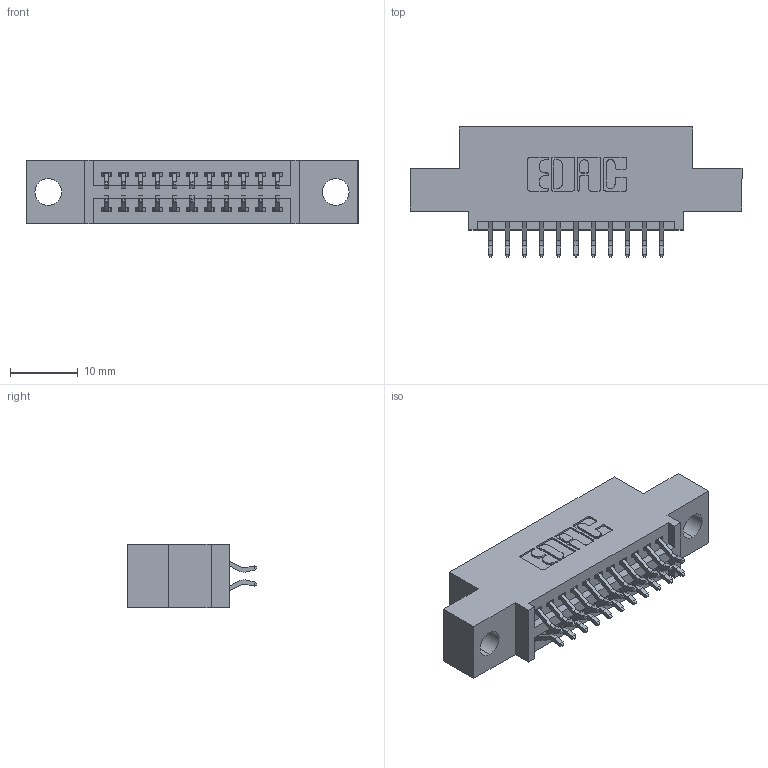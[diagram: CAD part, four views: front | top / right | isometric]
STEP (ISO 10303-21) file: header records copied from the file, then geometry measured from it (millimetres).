
FILE_DESCRIPTION (( 'STEP AP203' ), '1' );
FILE_NAME ('395-022-556-504.STEP', '2021-06-16T18:59:09', ( '' ), ( '' ), 'SwSTEP 2.0', 'SolidWorks 2020', '' );
FILE_SCHEMA (( 'CONFIG_CONTROL_DESIGN' ));
Length unit declared in the file: inch
Products named in the file (3): 345 Part_0.110 Offset - 0.156 Dia-TI; 395-022-556-504; 345-292-001_556 Tail
Assembly tree (23 placements, depth 2):
  395-022-556-504
    345 Part_0.110 Offset - 0.156 Dia-TI
    345-292-001_556 Tail  x22
Bounding box: 49.15 x 19.24 x 9.4 mm (x, y, z)
Volume: 4306.4 mm3; surface area: 5690.4 mm2
Topology: 23 solids, 23 shells, 1376 faces, 4063 edges, 2678 vertices
Faces by surface type: plane 912, cylinder 464
Entity records: 13575 total; most frequent: CARTESIAN_POINT 2326, ORIENTED_EDGE 2246, DIRECTION 2075, EDGE_CURVE 1123, VECTOR 939, LINE 939, VERTEX_POINT 746, AXIS2_PLACEMENT_3D 568
